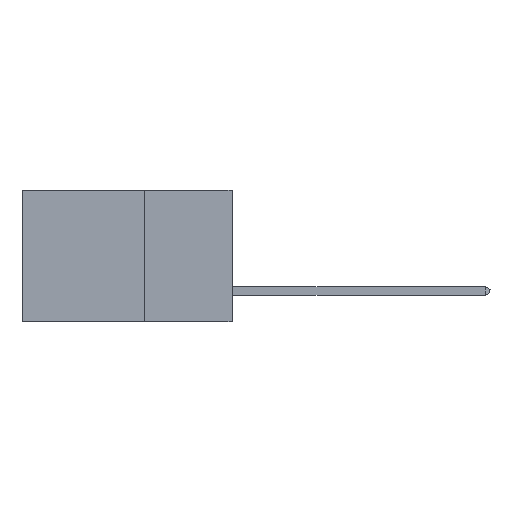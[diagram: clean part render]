
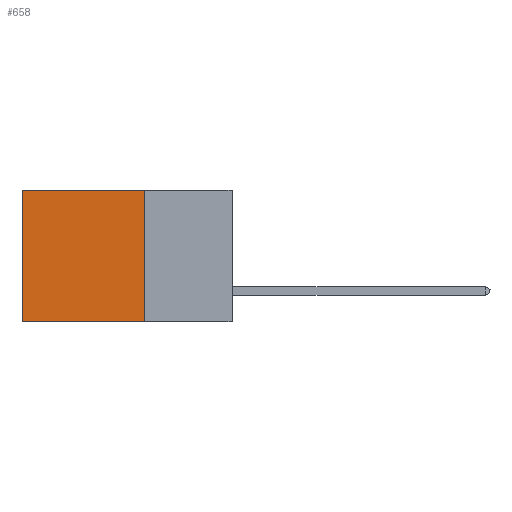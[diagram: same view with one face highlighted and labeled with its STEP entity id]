
A CAD part, left-side view. The second image highlights one B-rep face of the part: STEP entity #658.
In plain terms, the highlighted planar face has unit normal (-1, 0, 0).
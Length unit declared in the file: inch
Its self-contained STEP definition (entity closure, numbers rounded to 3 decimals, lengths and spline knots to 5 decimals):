
#216 = VECTOR ( 'NONE', #5294, 39.37008 ) ;
#320 = EDGE_CURVE ( 'NONE', #6853, #15305, #10668, .T. ) ;
#658 = ADVANCED_FACE ( 'NONE', ( #3411 ), #19739, .F. ) ;
#816 = DIRECTION ( 'NONE',  ( 0., 1., 0. ) ) ;
#1310 = VERTEX_POINT ( 'NONE', #3596 ) ;
#1405 = CARTESIAN_POINT ( 'NONE',  ( 0.2875, 0.25, -0.375 ) ) ;
#1697 = LINE ( 'NONE', #1405, #14725 ) ;
#2018 = CARTESIAN_POINT ( 'NONE',  ( 0.2875, 0.6, -0.375 ) ) ;
#2479 = VECTOR ( 'NONE', #816, 39.37008 ) ;
#2827 = EDGE_CURVE ( 'NONE', #1310, #15305, #3276, .T. ) ;
#3276 = LINE ( 'NONE', #12683, #2479 ) ;
#3411 = FACE_OUTER_BOUND ( 'NONE', #20964, .T. ) ;
#3596 = CARTESIAN_POINT ( 'NONE',  ( 0.2875, 0.25, -0.375 ) ) ;
#3626 = EDGE_CURVE ( 'NONE', #16153, #1310, #1697, .T. ) ;
#4671 = DIRECTION ( 'NONE',  ( 0., 0., -1. ) ) ;
#5294 = DIRECTION ( 'NONE',  ( 0., 0., -1. ) ) ;
#6853 = VERTEX_POINT ( 'NONE', #13522 ) ;
#7820 = VECTOR ( 'NONE', #19073, 39.37008 ) ;
#7915 = DIRECTION ( 'NONE',  ( 0., 0., -1. ) ) ;
#10668 = LINE ( 'NONE', #20636, #216 ) ;
#11429 = ORIENTED_EDGE ( 'NONE', *, *, #320, .T. ) ;
#12291 = AXIS2_PLACEMENT_3D ( 'NONE', #14668, #18115, #7915 ) ;
#12683 = CARTESIAN_POINT ( 'NONE',  ( 0.2875, 0.25, -0.375 ) ) ;
#12861 = LINE ( 'NONE', #14154, #7820 ) ;
#12931 = ORIENTED_EDGE ( 'NONE', *, *, #3626, .F. ) ;
#13522 = CARTESIAN_POINT ( 'NONE',  ( 0.2875, 0.6, 0. ) ) ;
#14154 = CARTESIAN_POINT ( 'NONE',  ( 0.2875, 0.25, 0. ) ) ;
#14668 = CARTESIAN_POINT ( 'NONE',  ( 0.2875, 0.25, -0.375 ) ) ;
#14725 = VECTOR ( 'NONE', #4671, 39.37008 ) ;
#15305 = VERTEX_POINT ( 'NONE', #2018 ) ;
#16153 = VERTEX_POINT ( 'NONE', #19025 ) ;
#18115 = DIRECTION ( 'NONE',  ( 1., 0., 0. ) ) ;
#19025 = CARTESIAN_POINT ( 'NONE',  ( 0.2875, 0.25, 0. ) ) ;
#19073 = DIRECTION ( 'NONE',  ( 0., 1., 0. ) ) ;
#19739 = PLANE ( 'NONE',  #12291 ) ;
#19949 = ORIENTED_EDGE ( 'NONE', *, *, #20884, .T. ) ;
#20636 = CARTESIAN_POINT ( 'NONE',  ( 0.2875, 0.6, -0.375 ) ) ;
#20884 = EDGE_CURVE ( 'NONE', #16153, #6853, #12861, .T. ) ;
#20902 = ORIENTED_EDGE ( 'NONE', *, *, #2827, .F. ) ;
#20964 = EDGE_LOOP ( 'NONE', ( #11429, #20902, #12931, #19949 ) ) ;
